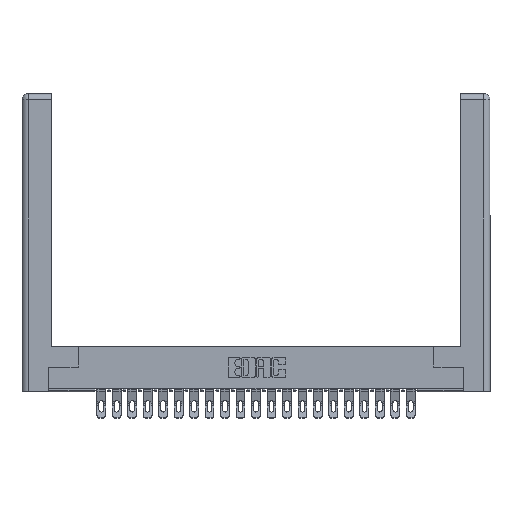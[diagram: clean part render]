
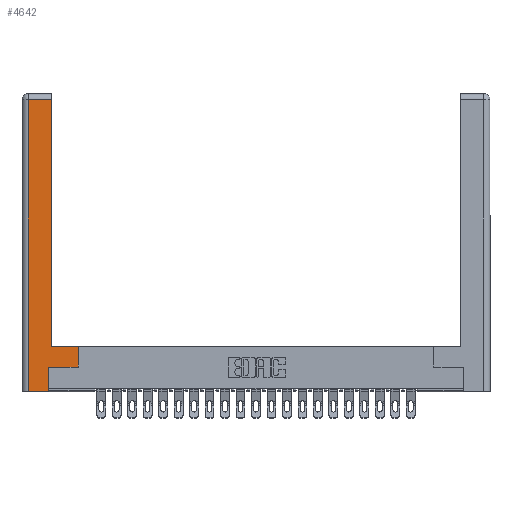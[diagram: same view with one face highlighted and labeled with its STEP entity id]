
A CAD part, top view. The second image highlights one B-rep face of the part: STEP entity #4642.
In plain terms, the highlighted planar face has unit normal (0, 0, 1).
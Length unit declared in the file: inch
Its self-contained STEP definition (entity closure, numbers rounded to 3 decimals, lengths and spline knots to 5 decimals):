
#113 = VECTOR ( 'NONE', #22909, 39.37008 ) ;
#925 = EDGE_CURVE ( 'NONE', #6049, #26520, #21455, .T. ) ;
#1849 = ORIENTED_EDGE ( 'NONE', *, *, #22439, .T. ) ;
#2178 = LINE ( 'NONE', #7364, #113 ) ;
#2402 = DIRECTION ( 'NONE',  ( -1., 0., 0. ) ) ;
#2813 = VERTEX_POINT ( 'NONE', #10910 ) ;
#2818 = VERTEX_POINT ( 'NONE', #22176 ) ;
#3536 = VERTEX_POINT ( 'NONE', #21923 ) ;
#3848 = DIRECTION ( 'NONE',  ( -1., 0., 0. ) ) ;
#3893 = CARTESIAN_POINT ( 'NONE',  ( 0.0615, 0., 0. ) ) ;
#4642 = ADVANCED_FACE ( 'NONE', ( #17457 ), #22091, .F. ) ;
#4682 = DIRECTION ( 'NONE',  ( 0., 1., 0. ) ) ;
#5203 = EDGE_CURVE ( 'NONE', #2813, #25250, #10205, .T. ) ;
#6049 = VERTEX_POINT ( 'NONE', #27470 ) ;
#6405 = VECTOR ( 'NONE', #15617, 39.37008 ) ;
#6411 = LINE ( 'NONE', #23805, #25721 ) ;
#6748 = EDGE_CURVE ( 'NONE', #3536, #8629, #2178, .T. ) ;
#7064 = DIRECTION ( 'NONE',  ( -1., 0., 0. ) ) ;
#7364 = CARTESIAN_POINT ( 'NONE',  ( 0.295, 3., 0. ) ) ;
#7426 = ORIENTED_EDGE ( 'NONE', *, *, #15807, .T. ) ;
#7536 = EDGE_LOOP ( 'NONE', ( #12818, #14193, #8660, #18475, #1849, #13220, #27098, #7426 ) ) ;
#8317 = DIRECTION ( 'NONE',  ( 0., -1., 0. ) ) ;
#8629 = VERTEX_POINT ( 'NONE', #24759 ) ;
#8660 = ORIENTED_EDGE ( 'NONE', *, *, #925, .T. ) ;
#8995 = VECTOR ( 'NONE', #8317, 39.37008 ) ;
#9645 = VECTOR ( 'NONE', #12535, 39.37008 ) ;
#9934 = CARTESIAN_POINT ( 'NONE',  ( 0.565, 0.45, 0. ) ) ;
#10205 = LINE ( 'NONE', #23102, #19856 ) ;
#10719 = EDGE_CURVE ( 'NONE', #8629, #6049, #26440, .T. ) ;
#10910 = CARTESIAN_POINT ( 'NONE',  ( 0.565, 0.245, 0. ) ) ;
#11223 = EDGE_CURVE ( 'NONE', #26520, #2818, #13689, .T. ) ;
#12535 = DIRECTION ( 'NONE',  ( 1., 0., 0. ) ) ;
#12818 = ORIENTED_EDGE ( 'NONE', *, *, #6748, .T. ) ;
#13220 = ORIENTED_EDGE ( 'NONE', *, *, #21081, .T. ) ;
#13233 = CARTESIAN_POINT ( 'NONE',  ( 0., 0., 0. ) ) ;
#13407 = CARTESIAN_POINT ( 'NONE',  ( 0.265, 0., 0. ) ) ;
#13689 = LINE ( 'NONE', #13407, #6405 ) ;
#13735 = VERTEX_POINT ( 'NONE', #24218 ) ;
#14193 = ORIENTED_EDGE ( 'NONE', *, *, #10719, .T. ) ;
#14550 = CARTESIAN_POINT ( 'NONE',  ( 0.565, 0.245, 0. ) ) ;
#15102 = LINE ( 'NONE', #20436, #21640 ) ;
#15121 = VECTOR ( 'NONE', #7064, 39.37008 ) ;
#15617 = DIRECTION ( 'NONE',  ( 1., 0., 0. ) ) ;
#15807 = EDGE_CURVE ( 'NONE', #25250, #3536, #6411, .T. ) ;
#16733 = DIRECTION ( 'NONE',  ( 0., 1., 0. ) ) ;
#17457 = FACE_OUTER_BOUND ( 'NONE', #7536, .T. ) ;
#17645 = DIRECTION ( 'NONE',  ( 0., 0., -1. ) ) ;
#18475 = ORIENTED_EDGE ( 'NONE', *, *, #11223, .T. ) ;
#19395 = AXIS2_PLACEMENT_3D ( 'NONE', #13233, #17645, #2402 ) ;
#19856 = VECTOR ( 'NONE', #16733, 39.37008 ) ;
#20436 = CARTESIAN_POINT ( 'NONE',  ( 0.265, 0.245, 0. ) ) ;
#21081 = EDGE_CURVE ( 'NONE', #13735, #2813, #22753, .T. ) ;
#21340 = CARTESIAN_POINT ( 'NONE',  ( 0.0615, 0., 0. ) ) ;
#21455 = LINE ( 'NONE', #3893, #8995 ) ;
#21640 = VECTOR ( 'NONE', #4682, 39.37008 ) ;
#21923 = CARTESIAN_POINT ( 'NONE',  ( 0.295, 0.45, 0. ) ) ;
#22091 = PLANE ( 'NONE',  #19395 ) ;
#22176 = CARTESIAN_POINT ( 'NONE',  ( 0.265, 0., 0. ) ) ;
#22439 = EDGE_CURVE ( 'NONE', #2818, #13735, #15102, .T. ) ;
#22753 = LINE ( 'NONE', #14550, #9645 ) ;
#22909 = DIRECTION ( 'NONE',  ( 0., 1., 0. ) ) ;
#23102 = CARTESIAN_POINT ( 'NONE',  ( 0.565, 0.45, 0. ) ) ;
#23805 = CARTESIAN_POINT ( 'NONE',  ( 0.295, 0.45, 0. ) ) ;
#24218 = CARTESIAN_POINT ( 'NONE',  ( 0.265, 0.245, 0. ) ) ;
#24759 = CARTESIAN_POINT ( 'NONE',  ( 0.295, 2.94, 0. ) ) ;
#24825 = CARTESIAN_POINT ( 'NONE',  ( 0.0615, 2.94, 0. ) ) ;
#25250 = VERTEX_POINT ( 'NONE', #9934 ) ;
#25721 = VECTOR ( 'NONE', #3848, 39.37008 ) ;
#26440 = LINE ( 'NONE', #24825, #15121 ) ;
#26520 = VERTEX_POINT ( 'NONE', #21340 ) ;
#27098 = ORIENTED_EDGE ( 'NONE', *, *, #5203, .T. ) ;
#27470 = CARTESIAN_POINT ( 'NONE',  ( 0.0615, 2.94, 0. ) ) ;
